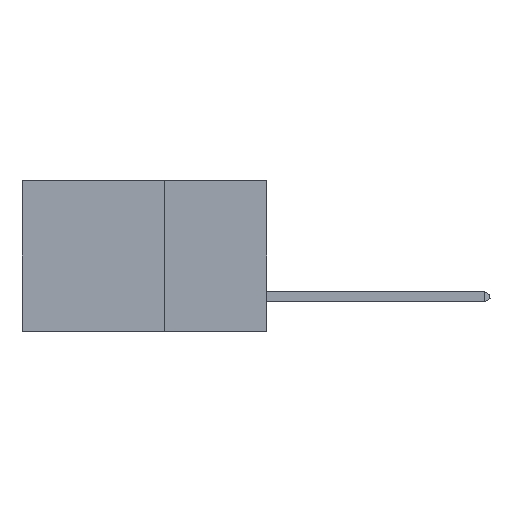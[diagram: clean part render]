
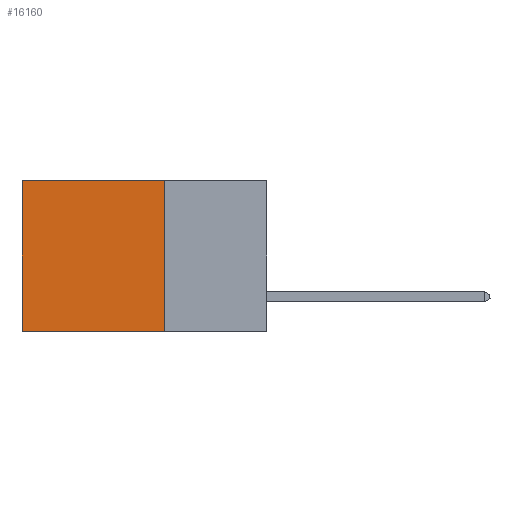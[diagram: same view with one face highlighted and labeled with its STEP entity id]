
A CAD part, left-side view. The second image highlights one B-rep face of the part: STEP entity #16160.
In plain terms, the highlighted planar face has unit normal (-1, 0, 0).
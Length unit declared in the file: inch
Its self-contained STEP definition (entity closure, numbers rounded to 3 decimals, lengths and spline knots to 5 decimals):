
#324 = DIRECTION ( 'NONE',  ( 0., 0., -1. ) ) ;
#1346 = DIRECTION ( 'NONE',  ( 0., 0., -1. ) ) ;
#2589 = EDGE_CURVE ( 'NONE', #33694, #29544, #5568, .T. ) ;
#3872 = LINE ( 'NONE', #16960, #13534 ) ;
#5568 = LINE ( 'NONE', #9943, #12904 ) ;
#8249 = ORIENTED_EDGE ( 'NONE', *, *, #39889, .F. ) ;
#9479 = CARTESIAN_POINT ( 'NONE',  ( 0.2875, 0.25, -0.37 ) ) ;
#9778 = LINE ( 'NONE', #25439, #15996 ) ;
#9943 = CARTESIAN_POINT ( 'NONE',  ( 0.2875, 0.25, 0. ) ) ;
#12904 = VECTOR ( 'NONE', #19089, 39.37008 ) ;
#13534 = VECTOR ( 'NONE', #27884, 39.37008 ) ;
#15623 = EDGE_CURVE ( 'NONE', #20549, #29291, #3872, .T. ) ;
#15996 = VECTOR ( 'NONE', #29210, 39.37008 ) ;
#16160 = ADVANCED_FACE ( 'NONE', ( #45839 ), #33887, .F. ) ;
#16960 = CARTESIAN_POINT ( 'NONE',  ( 0.2875, 0.25, -0.37 ) ) ;
#18978 = ORIENTED_EDGE ( 'NONE', *, *, #15623, .F. ) ;
#19089 = DIRECTION ( 'NONE',  ( 0., 1., 0. ) ) ;
#20110 = DIRECTION ( 'NONE',  ( 1., 0., 0. ) ) ;
#20549 = VERTEX_POINT ( 'NONE', #9479 ) ;
#20584 = EDGE_CURVE ( 'NONE', #29544, #29291, #9778, .T. ) ;
#21496 = CARTESIAN_POINT ( 'NONE',  ( 0.2875, 0.25, 0. ) ) ;
#25439 = CARTESIAN_POINT ( 'NONE',  ( 0.2875, 0.6, 0. ) ) ;
#26317 = CARTESIAN_POINT ( 'NONE',  ( 0.2875, 0.6, 0. ) ) ;
#27884 = DIRECTION ( 'NONE',  ( 0., 1., 0. ) ) ;
#28230 = CARTESIAN_POINT ( 'NONE',  ( 0.2875, 0.6, -0.37 ) ) ;
#28724 = CARTESIAN_POINT ( 'NONE',  ( 0.2875, 0.25, 0. ) ) ;
#29210 = DIRECTION ( 'NONE',  ( 0., 0., -1. ) ) ;
#29291 = VERTEX_POINT ( 'NONE', #28230 ) ;
#29544 = VERTEX_POINT ( 'NONE', #26317 ) ;
#30979 = VECTOR ( 'NONE', #324, 39.37008 ) ;
#33290 = LINE ( 'NONE', #28724, #30979 ) ;
#33694 = VERTEX_POINT ( 'NONE', #21496 ) ;
#33887 = PLANE ( 'NONE',  #45800 ) ;
#38736 = EDGE_LOOP ( 'NONE', ( #43936, #18978, #8249, #39186 ) ) ;
#39186 = ORIENTED_EDGE ( 'NONE', *, *, #2589, .T. ) ;
#39889 = EDGE_CURVE ( 'NONE', #33694, #20549, #33290, .T. ) ;
#41674 = CARTESIAN_POINT ( 'NONE',  ( 0.2875, 0.25, 0. ) ) ;
#43936 = ORIENTED_EDGE ( 'NONE', *, *, #20584, .T. ) ;
#45800 = AXIS2_PLACEMENT_3D ( 'NONE', #41674, #20110, #1346 ) ;
#45839 = FACE_OUTER_BOUND ( 'NONE', #38736, .T. ) ;
